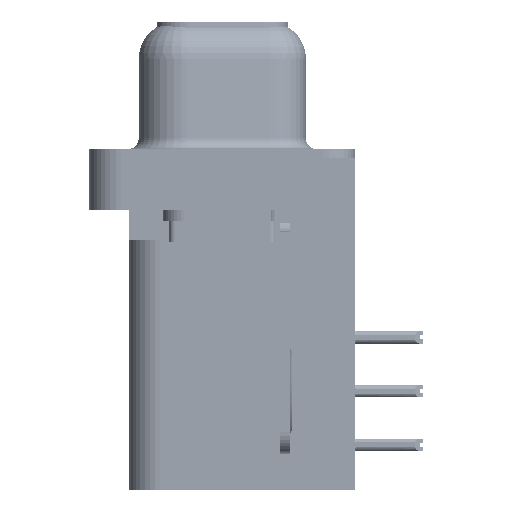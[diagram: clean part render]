
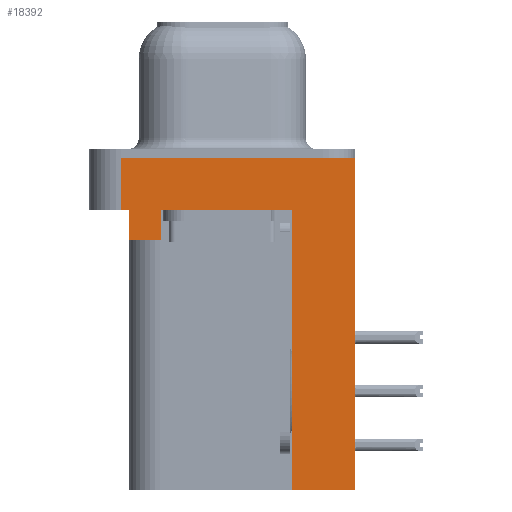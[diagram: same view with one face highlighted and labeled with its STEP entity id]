
A CAD part, left-side view. The second image highlights one B-rep face of the part: STEP entity #18392.
In plain terms, the highlighted planar face has unit normal (-1, 0, 0).
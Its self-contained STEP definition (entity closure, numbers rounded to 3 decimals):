
#297 = ORIENTED_EDGE ( 'NONE', *, *, #9584, .F. ) ;
#533 = CARTESIAN_POINT ( 'NONE',  ( -3., -6.275, -2.5 ) ) ;
#641 = LINE ( 'NONE', #8721, #10294 ) ;
#1915 = LINE ( 'NONE', #41308, #2221 ) ;
#2221 = VECTOR ( 'NONE', #19887, 1000. ) ;
#2397 = VECTOR ( 'NONE', #9180, 1000. ) ;
#2601 = LINE ( 'NONE', #27049, #2397 ) ;
#3876 = CARTESIAN_POINT ( 'NONE',  ( -3., -6.275, 0. ) ) ;
#4135 = CARTESIAN_POINT ( 'NONE',  ( -3., 4.775, -2.5 ) ) ;
#4775 = VERTEX_POINT ( 'NONE', #7163 ) ;
#5079 = DIRECTION ( 'NONE',  ( 0., 0., 1. ) ) ;
#5176 = CARTESIAN_POINT ( 'NONE',  ( -3., 4.425, -3.9 ) ) ;
#6820 = PLANE ( 'NONE',  #15690 ) ;
#6851 = EDGE_CURVE ( 'NONE', #42937, #41682, #19736, .T. ) ;
#7071 = EDGE_CURVE ( 'NONE', #33465, #41682, #18078, .T. ) ;
#7163 = CARTESIAN_POINT ( 'NONE',  ( -3., -3.295, -15.7 ) ) ;
#7470 = EDGE_CURVE ( 'NONE', #16491, #16778, #15732, .T. ) ;
#7540 = DIRECTION ( 'NONE',  ( 0., -1., 0. ) ) ;
#7923 = CARTESIAN_POINT ( 'NONE',  ( -3., 4.425, -3.9 ) ) ;
#8721 = CARTESIAN_POINT ( 'NONE',  ( -3., 4.425, -3.9 ) ) ;
#9117 = FACE_OUTER_BOUND ( 'NONE', #17664, .T. ) ;
#9180 = DIRECTION ( 'NONE',  ( 0., 0., 1. ) ) ;
#9584 = EDGE_CURVE ( 'NONE', #4775, #11031, #2601, .T. ) ;
#9623 = CARTESIAN_POINT ( 'NONE',  ( -3., 4.425, -2.5 ) ) ;
#10219 = VECTOR ( 'NONE', #18066, 1000. ) ;
#10294 = VECTOR ( 'NONE', #37335, 1000. ) ;
#10452 = CARTESIAN_POINT ( 'NONE',  ( -3., 2.895, -3.9 ) ) ;
#11031 = VERTEX_POINT ( 'NONE', #36733 ) ;
#11942 = VERTEX_POINT ( 'NONE', #24590 ) ;
#12379 = LINE ( 'NONE', #31772, #12473 ) ;
#12473 = VECTOR ( 'NONE', #38941, 1000. ) ;
#14054 = DIRECTION ( 'NONE',  ( 0., 0., 1. ) ) ;
#14741 = EDGE_CURVE ( 'NONE', #20467, #16778, #30750, .T. ) ;
#15355 = VECTOR ( 'NONE', #18658, 1000. ) ;
#15690 = AXIS2_PLACEMENT_3D ( 'NONE', #31896, #35432, #14054 ) ;
#15732 = LINE ( 'NONE', #533, #15355 ) ;
#16491 = VERTEX_POINT ( 'NONE', #26007 ) ;
#16778 = VERTEX_POINT ( 'NONE', #32255 ) ;
#17664 = EDGE_LOOP ( 'NONE', ( #32931, #40791, #27545, #25049, #39990, #24910, #25353, #297, #22227, #27228 ) ) ;
#17723 = VECTOR ( 'NONE', #41498, 1000. ) ;
#17937 = EDGE_CURVE ( 'NONE', #16491, #4775, #12379, .T. ) ;
#18066 = DIRECTION ( 'NONE',  ( 0., 0., 1. ) ) ;
#18078 = LINE ( 'NONE', #37963, #17723 ) ;
#18392 = ADVANCED_FACE ( 'NONE', ( #9117 ), #6820, .T. ) ;
#18658 = DIRECTION ( 'NONE',  ( 0., 0., 1. ) ) ;
#19657 = EDGE_CURVE ( 'NONE', #11942, #11031, #1915, .T. ) ;
#19736 = LINE ( 'NONE', #5176, #19781 ) ;
#19781 = VECTOR ( 'NONE', #5079, 1000. ) ;
#19887 = DIRECTION ( 'NONE',  ( 0., -1., 0. ) ) ;
#20467 = VERTEX_POINT ( 'NONE', #45984 ) ;
#22227 = ORIENTED_EDGE ( 'NONE', *, *, #17937, .F. ) ;
#22747 = CARTESIAN_POINT ( 'NONE',  ( -3., 4.775, -2.5 ) ) ;
#24590 = CARTESIAN_POINT ( 'NONE',  ( -3., 2.895, -2.5 ) ) ;
#24910 = ORIENTED_EDGE ( 'NONE', *, *, #44467, .T. ) ;
#25049 = ORIENTED_EDGE ( 'NONE', *, *, #6851, .F. ) ;
#25353 = ORIENTED_EDGE ( 'NONE', *, *, #19657, .T. ) ;
#25775 = EDGE_CURVE ( 'NONE', #33465, #20467, #37721, .T. ) ;
#26007 = CARTESIAN_POINT ( 'NONE',  ( -3., -6.275, -15.7 ) ) ;
#27049 = CARTESIAN_POINT ( 'NONE',  ( -3., -3.295, -15.7 ) ) ;
#27228 = ORIENTED_EDGE ( 'NONE', *, *, #7470, .T. ) ;
#27545 = ORIENTED_EDGE ( 'NONE', *, *, #7071, .T. ) ;
#28255 = VECTOR ( 'NONE', #32994, 1000. ) ;
#30551 = VECTOR ( 'NONE', #7540, 1000. ) ;
#30750 = LINE ( 'NONE', #3876, #30551 ) ;
#31772 = CARTESIAN_POINT ( 'NONE',  ( -3., -3.295, -15.7 ) ) ;
#31896 = CARTESIAN_POINT ( 'NONE',  ( -3., -6.275, -2.5 ) ) ;
#32255 = CARTESIAN_POINT ( 'NONE',  ( -3., -6.275, 0. ) ) ;
#32931 = ORIENTED_EDGE ( 'NONE', *, *, #14741, .F. ) ;
#32994 = DIRECTION ( 'NONE',  ( 0., 0., 1. ) ) ;
#33465 = VERTEX_POINT ( 'NONE', #22747 ) ;
#33476 = EDGE_CURVE ( 'NONE', #39615, #42937, #641, .T. ) ;
#35432 = DIRECTION ( 'NONE',  ( -1., 0., 0. ) ) ;
#36733 = CARTESIAN_POINT ( 'NONE',  ( -3., -3.295, -2.5 ) ) ;
#37335 = DIRECTION ( 'NONE',  ( 0., 1., 0. ) ) ;
#37664 = LINE ( 'NONE', #39529, #10219 ) ;
#37721 = LINE ( 'NONE', #4135, #28255 ) ;
#37963 = CARTESIAN_POINT ( 'NONE',  ( -3., -6.275, -2.5 ) ) ;
#38941 = DIRECTION ( 'NONE',  ( 0., 1., 0. ) ) ;
#39529 = CARTESIAN_POINT ( 'NONE',  ( -3., 2.895, -3.9 ) ) ;
#39615 = VERTEX_POINT ( 'NONE', #10452 ) ;
#39990 = ORIENTED_EDGE ( 'NONE', *, *, #33476, .F. ) ;
#40791 = ORIENTED_EDGE ( 'NONE', *, *, #25775, .F. ) ;
#41308 = CARTESIAN_POINT ( 'NONE',  ( -3., -6.275, -2.5 ) ) ;
#41498 = DIRECTION ( 'NONE',  ( 0., -1., 0. ) ) ;
#41682 = VERTEX_POINT ( 'NONE', #9623 ) ;
#42937 = VERTEX_POINT ( 'NONE', #7923 ) ;
#44467 = EDGE_CURVE ( 'NONE', #39615, #11942, #37664, .T. ) ;
#45984 = CARTESIAN_POINT ( 'NONE',  ( -3., 4.775, 0. ) ) ;
